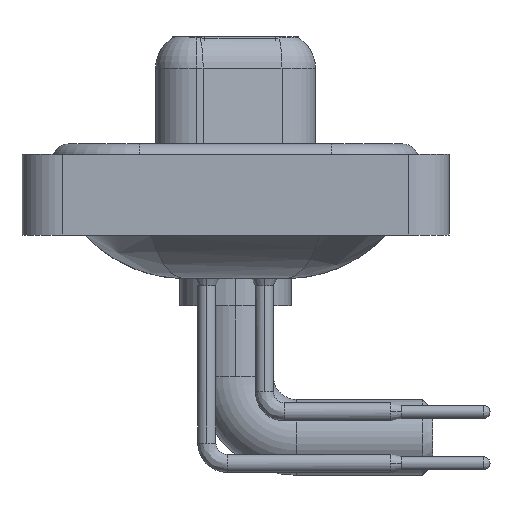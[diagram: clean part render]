
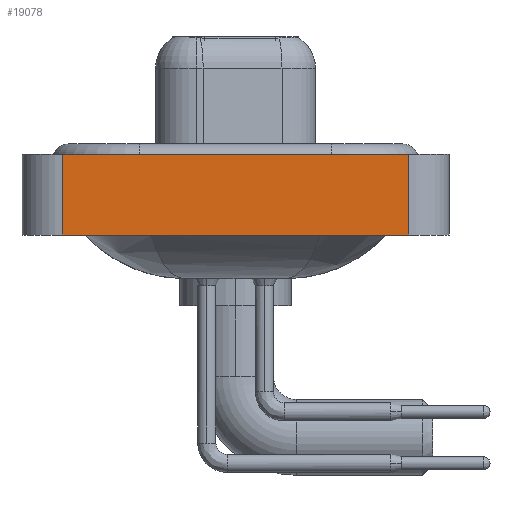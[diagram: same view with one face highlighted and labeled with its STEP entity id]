
A CAD part, left-side view. The second image highlights one B-rep face of the part: STEP entity #19078.
In plain terms, the highlighted planar face has unit normal (-1, 0, 0).
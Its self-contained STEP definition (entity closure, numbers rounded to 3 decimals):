
#228 = VECTOR ( 'NONE', #19824, 1000. ) ;
#268 = CARTESIAN_POINT ( 'NONE',  ( -7.3, -8.55, -3.6 ) ) ;
#283 = VECTOR ( 'NONE', #15072, 1000. ) ;
#1122 = VECTOR ( 'NONE', #15018, 1000. ) ;
#1206 = ORIENTED_EDGE ( 'NONE', *, *, #18465, .F. ) ;
#1225 = CARTESIAN_POINT ( 'NONE',  ( -7.3, -8.55, 0.4 ) ) ;
#1981 = CARTESIAN_POINT ( 'NONE',  ( -7.3, -8.55, -3.6 ) ) ;
#3380 = VERTEX_POINT ( 'NONE', #17704 ) ;
#4258 = VECTOR ( 'NONE', #7703, 1000. ) ;
#4603 = LINE ( 'NONE', #1225, #4258 ) ;
#4842 = CARTESIAN_POINT ( 'NONE',  ( -7.3, -8.55, 0.4 ) ) ;
#7415 = FACE_OUTER_BOUND ( 'NONE', #9848, .T. ) ;
#7703 = DIRECTION ( 'NONE',  ( 0., -1., 0. ) ) ;
#9774 = CARTESIAN_POINT ( 'NONE',  ( -7.3, 8.55, 0.4 ) ) ;
#9848 = EDGE_LOOP ( 'NONE', ( #19592, #1206, #17135, #19644 ) ) ;
#10281 = VERTEX_POINT ( 'NONE', #9774 ) ;
#10717 = PLANE ( 'NONE',  #11885 ) ;
#11885 = AXIS2_PLACEMENT_3D ( 'NONE', #1981, #17596, #14116 ) ;
#11897 = CARTESIAN_POINT ( 'NONE',  ( -7.3, 8.55, -3.6 ) ) ;
#12198 = CARTESIAN_POINT ( 'NONE',  ( -7.3, -8.55, -3.6 ) ) ;
#12400 = EDGE_CURVE ( 'NONE', #3380, #10281, #16998, .T. ) ;
#12932 = LINE ( 'NONE', #14637, #228 ) ;
#13314 = LINE ( 'NONE', #268, #1122 ) ;
#13885 = VERTEX_POINT ( 'NONE', #4842 ) ;
#14116 = DIRECTION ( 'NONE',  ( 0., 0., 1. ) ) ;
#14281 = VERTEX_POINT ( 'NONE', #12198 ) ;
#14637 = CARTESIAN_POINT ( 'NONE',  ( -7.3, -8.55, -3.6 ) ) ;
#14942 = EDGE_CURVE ( 'NONE', #14281, #13885, #12932, .T. ) ;
#15018 = DIRECTION ( 'NONE',  ( 0., -1., 0. ) ) ;
#15072 = DIRECTION ( 'NONE',  ( 0., 0., 1. ) ) ;
#16998 = LINE ( 'NONE', #11897, #283 ) ;
#17135 = ORIENTED_EDGE ( 'NONE', *, *, #12400, .F. ) ;
#17596 = DIRECTION ( 'NONE',  ( -1., 0., 0. ) ) ;
#17690 = EDGE_CURVE ( 'NONE', #3380, #14281, #13314, .T. ) ;
#17704 = CARTESIAN_POINT ( 'NONE',  ( -7.3, 8.55, -3.6 ) ) ;
#18465 = EDGE_CURVE ( 'NONE', #10281, #13885, #4603, .T. ) ;
#19078 = ADVANCED_FACE ( 'NONE', ( #7415 ), #10717, .T. ) ;
#19592 = ORIENTED_EDGE ( 'NONE', *, *, #14942, .T. ) ;
#19644 = ORIENTED_EDGE ( 'NONE', *, *, #17690, .T. ) ;
#19824 = DIRECTION ( 'NONE',  ( 0., 0., 1. ) ) ;
